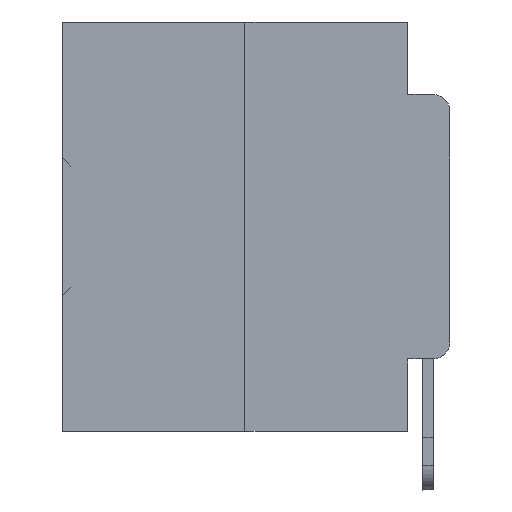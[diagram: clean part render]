
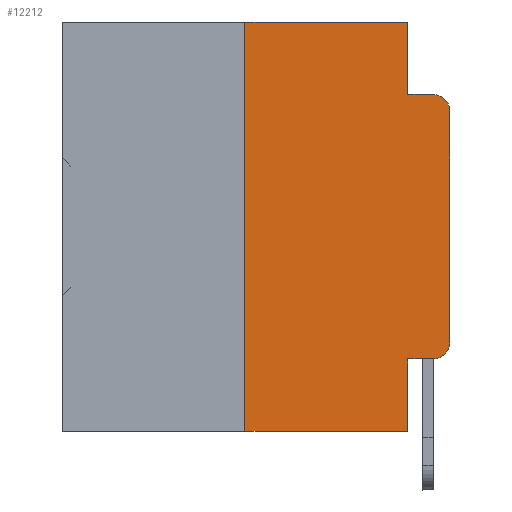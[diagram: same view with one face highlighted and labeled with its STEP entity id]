
A CAD part, left-side view. The second image highlights one B-rep face of the part: STEP entity #12212.
In plain terms, the highlighted planar face has unit normal (-1, 0, 0).
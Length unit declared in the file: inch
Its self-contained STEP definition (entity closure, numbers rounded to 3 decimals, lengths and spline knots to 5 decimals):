
#244 = VERTEX_POINT ( 'NONE', #4566 ) ;
#383 = DIRECTION ( 'NONE',  ( 0., 0., 1. ) ) ;
#1855 = VECTOR ( 'NONE', #383, 39.37008 ) ;
#1860 = CARTESIAN_POINT ( 'NONE',  ( 0., 0.473, 0. ) ) ;
#1918 = CARTESIAN_POINT ( 'NONE',  ( 0., 0.25, 0. ) ) ;
#2621 = DIRECTION ( 'NONE',  ( 0., 0., -1. ) ) ;
#2770 = EDGE_CURVE ( 'NONE', #37169, #3223, #26452, .T. ) ;
#2874 = EDGE_CURVE ( 'NONE', #17329, #7327, #27788, .T. ) ;
#3044 = ORIENTED_EDGE ( 'NONE', *, *, #7395, .F. ) ;
#3223 = VERTEX_POINT ( 'NONE', #29490 ) ;
#3414 = VECTOR ( 'NONE', #22720, 39.37008 ) ;
#3682 = VERTEX_POINT ( 'NONE', #36665 ) ;
#4566 = CARTESIAN_POINT ( 'NONE',  ( 0., 0.051, -0.4115 ) ) ;
#5022 = DIRECTION ( 'NONE',  ( 1., 0., 0. ) ) ;
#5227 = CARTESIAN_POINT ( 'NONE',  ( 0., 0.473, -0.5 ) ) ;
#5287 = DIRECTION ( 'NONE',  ( 0., 0., -1. ) ) ;
#5431 = ORIENTED_EDGE ( 'NONE', *, *, #2770, .T. ) ;
#5485 = DIRECTION ( 'NONE',  ( 0., -1., 0. ) ) ;
#5489 = CARTESIAN_POINT ( 'NONE',  ( 0., 0.25, 0. ) ) ;
#7327 = VERTEX_POINT ( 'NONE', #1918 ) ;
#7395 = EDGE_CURVE ( 'NONE', #13798, #3223, #26586, .T. ) ;
#7421 = LINE ( 'NONE', #5227, #16714 ) ;
#8325 = DIRECTION ( 'NONE',  ( 0., -1., 0. ) ) ;
#8870 = DIRECTION ( 'NONE',  ( 0., 0., -1. ) ) ;
#10110 = VERTEX_POINT ( 'NONE', #25315 ) ;
#10262 = EDGE_CURVE ( 'NONE', #7327, #10110, #31671, .T. ) ;
#10897 = EDGE_LOOP ( 'NONE', ( #31694, #5431, #3044, #37569, #30729, #14593, #24216, #35797, #12002, #28671 ) ) ;
#11039 = CARTESIAN_POINT ( 'NONE',  ( 0., 0.051, -0.5 ) ) ;
#11112 = CARTESIAN_POINT ( 'NONE',  ( 0., 0., -0.3915 ) ) ;
#11686 = CARTESIAN_POINT ( 'NONE',  ( 0., 0., 0. ) ) ;
#12002 = ORIENTED_EDGE ( 'NONE', *, *, #20726, .T. ) ;
#12212 = ADVANCED_FACE ( 'NONE', ( #33333 ), #37552, .F. ) ;
#12514 = CARTESIAN_POINT ( 'NONE',  ( 0., 0., -0.1085 ) ) ;
#12612 = VECTOR ( 'NONE', #37981, 39.37008 ) ;
#13798 = VERTEX_POINT ( 'NONE', #34536 ) ;
#14142 = DIRECTION ( 'NONE',  ( -1., 0., 0. ) ) ;
#14593 = ORIENTED_EDGE ( 'NONE', *, *, #2874, .F. ) ;
#15171 = VECTOR ( 'NONE', #36146, 39.37008 ) ;
#16089 = LINE ( 'NONE', #21411, #15171 ) ;
#16397 = VECTOR ( 'NONE', #19938, 39.37008 ) ;
#16714 = VECTOR ( 'NONE', #8325, 39.37008 ) ;
#17329 = VERTEX_POINT ( 'NONE', #18262 ) ;
#17751 = DIRECTION ( 'NONE',  ( -1., 0., 0. ) ) ;
#18262 = CARTESIAN_POINT ( 'NONE',  ( 0., 0.25, -0.5 ) ) ;
#18599 = LINE ( 'NONE', #11686, #12612 ) ;
#19612 = VERTEX_POINT ( 'NONE', #11039 ) ;
#19713 = CARTESIAN_POINT ( 'NONE',  ( 0., 0.02, -0.3915 ) ) ;
#19749 = EDGE_CURVE ( 'NONE', #31565, #37169, #18599, .T. ) ;
#19791 = CARTESIAN_POINT ( 'NONE',  ( 0., 0.473, 0. ) ) ;
#19938 = DIRECTION ( 'NONE',  ( 0., -1., 0. ) ) ;
#20712 = EDGE_CURVE ( 'NONE', #17329, #19612, #7421, .T. ) ;
#20726 = EDGE_CURVE ( 'NONE', #244, #3682, #29183, .T. ) ;
#21411 = CARTESIAN_POINT ( 'NONE',  ( 0., 0.051, 0. ) ) ;
#22670 = DIRECTION ( 'NONE',  ( 0., 0., -1. ) ) ;
#22702 = CARTESIAN_POINT ( 'NONE',  ( 0., 0.051, -0.4115 ) ) ;
#22720 = DIRECTION ( 'NONE',  ( 0., -1., 0. ) ) ;
#23471 = CARTESIAN_POINT ( 'NONE',  ( 0., 0.02, -0.1085 ) ) ;
#24216 = ORIENTED_EDGE ( 'NONE', *, *, #20712, .T. ) ;
#25315 = CARTESIAN_POINT ( 'NONE',  ( 0., 0.051, 0. ) ) ;
#25839 = VECTOR ( 'NONE', #8870, 39.37008 ) ;
#26314 = LINE ( 'NONE', #35528, #25839 ) ;
#26452 = CIRCLE ( 'NONE', #26735, 0.02 ) ;
#26586 = LINE ( 'NONE', #31668, #16397 ) ;
#26735 = AXIS2_PLACEMENT_3D ( 'NONE', #23471, #17751, #2621 ) ;
#27171 = AXIS2_PLACEMENT_3D ( 'NONE', #19791, #5022, #5287 ) ;
#27605 = EDGE_CURVE ( 'NONE', #3682, #31565, #36301, .T. ) ;
#27788 = LINE ( 'NONE', #5489, #1855 ) ;
#28671 = ORIENTED_EDGE ( 'NONE', *, *, #27605, .T. ) ;
#29183 = LINE ( 'NONE', #22702, #37580 ) ;
#29490 = CARTESIAN_POINT ( 'NONE',  ( 0., 0.02, -0.0885 ) ) ;
#30729 = ORIENTED_EDGE ( 'NONE', *, *, #10262, .F. ) ;
#31507 = AXIS2_PLACEMENT_3D ( 'NONE', #19713, #14142, #22670 ) ;
#31565 = VERTEX_POINT ( 'NONE', #11112 ) ;
#31668 = CARTESIAN_POINT ( 'NONE',  ( 0., 0.051, -0.0885 ) ) ;
#31671 = LINE ( 'NONE', #1860, #3414 ) ;
#31694 = ORIENTED_EDGE ( 'NONE', *, *, #19749, .T. ) ;
#33333 = FACE_OUTER_BOUND ( 'NONE', #10897, .T. ) ;
#34354 = EDGE_CURVE ( 'NONE', #244, #19612, #26314, .T. ) ;
#34472 = EDGE_CURVE ( 'NONE', #10110, #13798, #16089, .T. ) ;
#34536 = CARTESIAN_POINT ( 'NONE',  ( 0., 0.051, -0.0885 ) ) ;
#35528 = CARTESIAN_POINT ( 'NONE',  ( 0., 0.051, 0. ) ) ;
#35797 = ORIENTED_EDGE ( 'NONE', *, *, #34354, .F. ) ;
#36146 = DIRECTION ( 'NONE',  ( 0., 0., -1. ) ) ;
#36301 = CIRCLE ( 'NONE', #31507, 0.02 ) ;
#36665 = CARTESIAN_POINT ( 'NONE',  ( 0., 0.02, -0.4115 ) ) ;
#37169 = VERTEX_POINT ( 'NONE', #12514 ) ;
#37552 = PLANE ( 'NONE',  #27171 ) ;
#37569 = ORIENTED_EDGE ( 'NONE', *, *, #34472, .F. ) ;
#37580 = VECTOR ( 'NONE', #5485, 39.37008 ) ;
#37981 = DIRECTION ( 'NONE',  ( 0., 0., 1. ) ) ;
